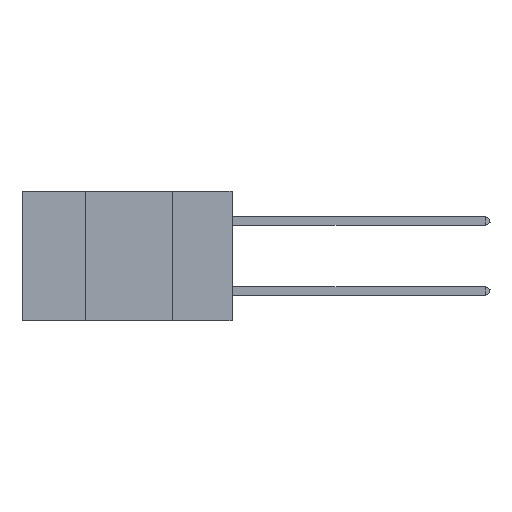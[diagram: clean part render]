
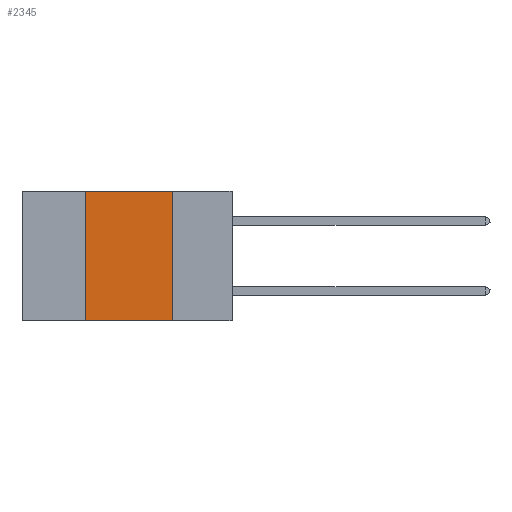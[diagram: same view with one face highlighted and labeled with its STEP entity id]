
A CAD part, left-side view. The second image highlights one B-rep face of the part: STEP entity #2345.
In plain terms, the highlighted planar face has unit normal (-1, 0, 0).
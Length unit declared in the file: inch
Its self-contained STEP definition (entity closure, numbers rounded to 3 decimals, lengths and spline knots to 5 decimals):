
#64 = LINE ( 'NONE', #12069, #2544 ) ;
#602 = VERTEX_POINT ( 'NONE', #5404 ) ;
#1366 = CARTESIAN_POINT ( 'NONE',  ( 0., 0.42, -0.37 ) ) ;
#1968 = VERTEX_POINT ( 'NONE', #5892 ) ;
#2096 = DIRECTION ( 'NONE',  ( 0., -1., 0. ) ) ;
#2254 = LINE ( 'NONE', #12538, #11945 ) ;
#2255 = LINE ( 'NONE', #8011, #10034 ) ;
#2273 = DIRECTION ( 'NONE',  ( 0., 0., -1. ) ) ;
#2345 = ADVANCED_FACE ( 'NONE', ( #5203 ), #11002, .F. ) ;
#2397 = ORIENTED_EDGE ( 'NONE', *, *, #7186, .F. ) ;
#2544 = VECTOR ( 'NONE', #6387, 39.37008 ) ;
#2559 = CARTESIAN_POINT ( 'NONE',  ( 0., 0.17, 0. ) ) ;
#2686 = ORIENTED_EDGE ( 'NONE', *, *, #6544, .F. ) ;
#2720 = ORIENTED_EDGE ( 'NONE', *, *, #11709, .F. ) ;
#2801 = DIRECTION ( 'NONE',  ( 0., 0., -1. ) ) ;
#2921 = ORIENTED_EDGE ( 'NONE', *, *, #8422, .T. ) ;
#4985 = DIRECTION ( 'NONE',  ( 0., 0., 1. ) ) ;
#5203 = FACE_OUTER_BOUND ( 'NONE', #9485, .T. ) ;
#5404 = CARTESIAN_POINT ( 'NONE',  ( 0., 0.17, -0.37 ) ) ;
#5765 = LINE ( 'NONE', #8630, #8561 ) ;
#5892 = CARTESIAN_POINT ( 'NONE',  ( 0., 0.42, 0. ) ) ;
#6272 = CARTESIAN_POINT ( 'NONE',  ( 0., 0.6, 0. ) ) ;
#6387 = DIRECTION ( 'NONE',  ( 0., -1., 0. ) ) ;
#6544 = EDGE_CURVE ( 'NONE', #6924, #602, #5765, .T. ) ;
#6868 = VERTEX_POINT ( 'NONE', #1366 ) ;
#6924 = VERTEX_POINT ( 'NONE', #2559 ) ;
#6975 = AXIS2_PLACEMENT_3D ( 'NONE', #6272, #8163, #2273 ) ;
#7186 = EDGE_CURVE ( 'NONE', #6868, #1968, #2254, .T. ) ;
#8011 = CARTESIAN_POINT ( 'NONE',  ( 0., 0.6, 0. ) ) ;
#8163 = DIRECTION ( 'NONE',  ( 1., 0., 0. ) ) ;
#8422 = EDGE_CURVE ( 'NONE', #6868, #602, #64, .T. ) ;
#8561 = VECTOR ( 'NONE', #2801, 39.37008 ) ;
#8630 = CARTESIAN_POINT ( 'NONE',  ( 0., 0.17, 0. ) ) ;
#9485 = EDGE_LOOP ( 'NONE', ( #2686, #2720, #2397, #2921 ) ) ;
#10034 = VECTOR ( 'NONE', #2096, 39.37008 ) ;
#11002 = PLANE ( 'NONE',  #6975 ) ;
#11709 = EDGE_CURVE ( 'NONE', #1968, #6924, #2255, .T. ) ;
#11945 = VECTOR ( 'NONE', #4985, 39.37008 ) ;
#12069 = CARTESIAN_POINT ( 'NONE',  ( 0., 0.6, -0.37 ) ) ;
#12538 = CARTESIAN_POINT ( 'NONE',  ( 0., 0.42, 0. ) ) ;
